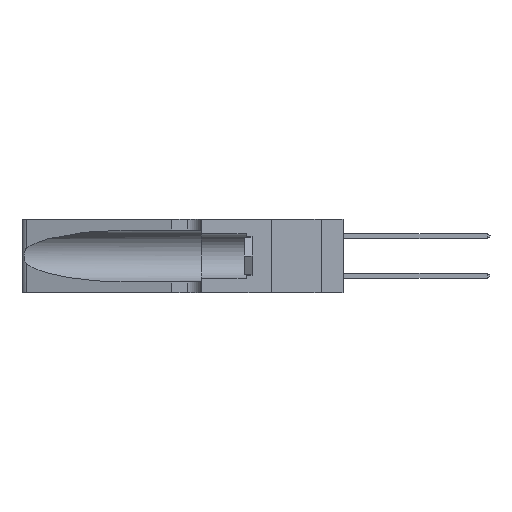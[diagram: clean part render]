
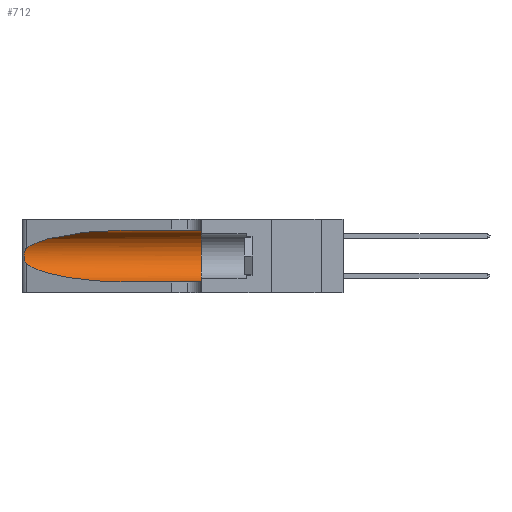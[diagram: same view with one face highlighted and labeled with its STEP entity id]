
A CAD part, left-side view. The second image highlights one B-rep face of the part: STEP entity #712.
In plain terms, the highlighted cylindrical face has radius 3.308 mm (diameter 6.617 mm), a partial arc.
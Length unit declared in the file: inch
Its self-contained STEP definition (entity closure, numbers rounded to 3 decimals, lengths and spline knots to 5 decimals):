
#203 = DIRECTION ( 'NONE',  ( 0., 0., 1. ) ) ;
#317 = CARTESIAN_POINT ( 'NONE',  ( 0.1305, 1.61858, 0.05475 ) ) ;
#670 = CARTESIAN_POINT ( 'NONE',  ( 0.1305, 0.72297, 0.05475 ) ) ;
#712 = ADVANCED_FACE ( 'NONE', ( #34175 ), #19496, .F. ) ;
#745 = CARTESIAN_POINT ( 'NONE',  ( 0.26075, 1.23896, 0.178 ) ) ;
#1513 = CARTESIAN_POINT ( 'NONE',  ( 0.18966, 0.96281, 0.31525 ) ) ;
#2999 = EDGE_LOOP ( 'NONE', ( #28928, #7705, #30658, #16809, #24180, #33230 ) ) ;
#3577 = CARTESIAN_POINT ( 'NONE',  ( 0.25856, 1.23593, 0.16098 ) ) ;
#4374 = EDGE_CURVE ( 'NONE', #12903, #12092, #25355, .T. ) ;
#4649 = VERTEX_POINT ( 'NONE', #26464 ) ;
#6380 = CARTESIAN_POINT ( 'NONE',  ( 0.25639, 1.23186, 0.15144 ) ) ;
#7705 = ORIENTED_EDGE ( 'NONE', *, *, #34043, .T. ) ;
#7961 = VERTEX_POINT ( 'NONE', #23451 ) ;
#7981 = DIRECTION ( 'NONE',  ( 0., 0., -1. ) ) ;
#9179 = CARTESIAN_POINT ( 'NONE',  ( 0.25487, 1.22718, 0.14631 ) ) ;
#9831 = LINE ( 'NONE', #27668, #31043 ) ;
#9954 = CARTESIAN_POINT ( 'NONE',  ( 0.2373, 1.15595, 0.28018 ) ) ;
#10626 = VECTOR ( 'NONE', #17014, 39.37008 ) ;
#11808 = CARTESIAN_POINT ( 'NONE',  ( 0.2373, 1.15595, 0.08982 ) ) ;
#11874 = CARTESIAN_POINT ( 'NONE',  ( 0.25639, 1.23184, 0.21858 ) ) ;
#12092 = VERTEX_POINT ( 'NONE', #22682 ) ;
#12903 = VERTEX_POINT ( 'NONE', #28662 ) ;
#14533 = CARTESIAN_POINT ( 'NONE',  ( 0.25555, 1.22994, 0.2215 ) ) ;
#14656 = CARTESIAN_POINT ( 'NONE',  ( 0.25854, 1.2359, 0.20912 ) ) ;
#16583 = VERTEX_POINT ( 'NONE', #19287 ) ;
#16809 = ORIENTED_EDGE ( 'NONE', *, *, #4374, .T. ) ;
#16904 = DIRECTION ( 'NONE',  ( 0., 1., 0. ) ) ;
#16987 = EDGE_CURVE ( 'NONE', #28978, #4649, #34952, .T. ) ;
#17014 = DIRECTION ( 'NONE',  ( 0., -1., 0. ) ) ;
#17357 = CARTESIAN_POINT ( 'NONE',  ( 0.18966, 0.96281, 0.05475 ) ) ;
#17419 = CARTESIAN_POINT ( 'NONE',  ( 0.26075, 1.23896, 0.19203 ) ) ;
#18357 = EDGE_CURVE ( 'NONE', #16583, #12092, #28816, .T. ) ;
#18556 = CARTESIAN_POINT ( 'NONE',  ( 0.1305, 0.72297, 0.31525 ) ) ;
#19287 = CARTESIAN_POINT ( 'NONE',  ( 0.1305, 0.35, 0.31525 ) ) ;
#19496 = CYLINDRICAL_SURFACE ( 'NONE', #35309, 0.13025 ) ;
#20094 = CARTESIAN_POINT ( 'NONE',  ( 0.25487, 1.22718, 0.22369 ) ) ;
#20204 = CARTESIAN_POINT ( 'NONE',  ( 0.26017, 1.23833, 0.17102 ) ) ;
#20964 = CARTESIAN_POINT ( 'NONE',  ( 0.1305, 0.72297, 0.31525 ) ) ;
#22150 =( BOUNDED_CURVE ( )  B_SPLINE_CURVE ( 3, ( #31149, #11808, #17357, #670 ),
 .UNSPECIFIED., .F., .T. ) 
 B_SPLINE_CURVE_WITH_KNOTS ( ( 4, 4 ),
 ( 3.44316, 4.71239 ),
 .UNSPECIFIED. ) 
 CURVE ( )  GEOMETRIC_REPRESENTATION_ITEM ( )  RATIONAL_B_SPLINE_CURVE ( ( 1., 0.87, 0.87, 1. ) ) 
 REPRESENTATION_ITEM ( '' )  );
#22682 = CARTESIAN_POINT ( 'NONE',  ( 0.1305, 0.35, 0.05475 ) ) ;
#23008 = CARTESIAN_POINT ( 'NONE',  ( 0.25789, 1.23486, 0.15765 ) ) ;
#23451 = CARTESIAN_POINT ( 'NONE',  ( 0.25487, 1.22718, 0.14631 ) ) ;
#24011 = AXIS2_PLACEMENT_3D ( 'NONE', #33437, #16904, #203 ) ;
#24180 = ORIENTED_EDGE ( 'NONE', *, *, #18357, .F. ) ;
#25355 = LINE ( 'NONE', #317, #10626 ) ;
#25788 = CARTESIAN_POINT ( 'NONE',  ( 0.25555, 1.22993, 0.14849 ) ) ;
#25917 = B_SPLINE_CURVE_WITH_KNOTS ( 'NONE', 3,
 ( #20094, #14533, #11874, #31211, #14656, #33953, #17419, #745, #20204, #3577, #23008, #6380, #25788, #9179 ),
 .UNSPECIFIED., .F., .F.,
 ( 4, 2, 2, 2, 2, 2, 4 ),
 ( 0., 0.00027, 0.00053, 0.00107, 0.0016, 0.00187, 0.00214 ),
 .UNSPECIFIED. ) ;
#26355 = EDGE_CURVE ( 'NONE', #7961, #12903, #22150, .T. ) ;
#26464 = CARTESIAN_POINT ( 'NONE',  ( 0.25487, 1.22718, 0.22369 ) ) ;
#27343 = DIRECTION ( 'NONE',  ( 0., -1., 0. ) ) ;
#27668 = CARTESIAN_POINT ( 'NONE',  ( 0.1305, 1.61858, 0.31525 ) ) ;
#28662 = CARTESIAN_POINT ( 'NONE',  ( 0.1305, 0.72297, 0.05475 ) ) ;
#28816 = CIRCLE ( 'NONE', #24011, 0.13025 ) ;
#28928 = ORIENTED_EDGE ( 'NONE', *, *, #16987, .T. ) ;
#28978 = VERTEX_POINT ( 'NONE', #18556 ) ;
#29297 = CARTESIAN_POINT ( 'NONE',  ( 0.25487, 1.22718, 0.22369 ) ) ;
#29884 = CARTESIAN_POINT ( 'NONE',  ( 0.1305, 1.61858, 0.185 ) ) ;
#29901 = EDGE_CURVE ( 'NONE', #28978, #16583, #9831, .T. ) ;
#30455 = DIRECTION ( 'NONE',  ( 0., -1., 0. ) ) ;
#30658 = ORIENTED_EDGE ( 'NONE', *, *, #26355, .T. ) ;
#31043 = VECTOR ( 'NONE', #30455, 39.37008 ) ;
#31149 = CARTESIAN_POINT ( 'NONE',  ( 0.25487, 1.22718, 0.14631 ) ) ;
#31211 = CARTESIAN_POINT ( 'NONE',  ( 0.25787, 1.23484, 0.2124 ) ) ;
#33230 = ORIENTED_EDGE ( 'NONE', *, *, #29901, .F. ) ;
#33437 = CARTESIAN_POINT ( 'NONE',  ( 0.1305, 0.35, 0.185 ) ) ;
#33953 = CARTESIAN_POINT ( 'NONE',  ( 0.26018, 1.23835, 0.19895 ) ) ;
#34043 = EDGE_CURVE ( 'NONE', #4649, #7961, #25917, .T. ) ;
#34175 = FACE_OUTER_BOUND ( 'NONE', #2999, .T. ) ;
#34952 =( BOUNDED_CURVE ( )  B_SPLINE_CURVE ( 3, ( #20964, #1513, #9954, #29297 ),
 .UNSPECIFIED., .F., .T. ) 
 B_SPLINE_CURVE_WITH_KNOTS ( ( 4, 4 ),
 ( 1.5708, 2.84003 ),
 .UNSPECIFIED. ) 
 CURVE ( )  GEOMETRIC_REPRESENTATION_ITEM ( )  RATIONAL_B_SPLINE_CURVE ( ( 1., 0.87, 0.87, 1. ) ) 
 REPRESENTATION_ITEM ( '' )  );
#35309 = AXIS2_PLACEMENT_3D ( 'NONE', #29884, #27343, #7981 ) ;
